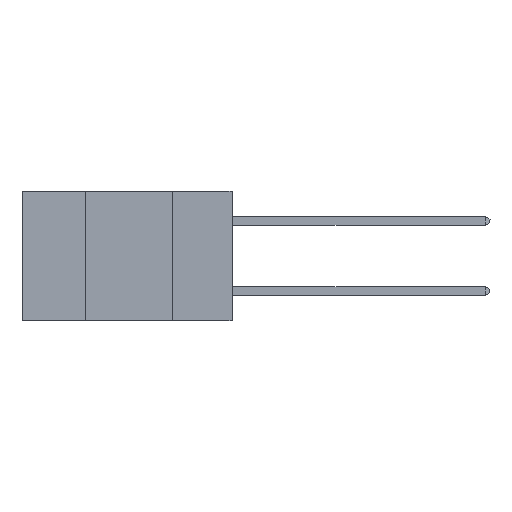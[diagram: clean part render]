
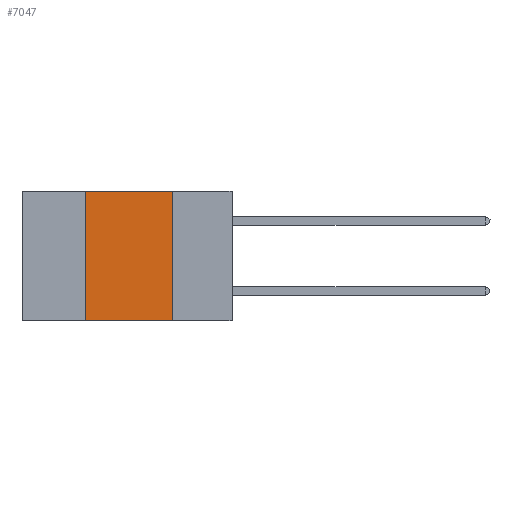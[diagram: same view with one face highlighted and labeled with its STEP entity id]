
A CAD part, left-side view. The second image highlights one B-rep face of the part: STEP entity #7047.
In plain terms, the highlighted planar face has unit normal (-1, 0, 0).
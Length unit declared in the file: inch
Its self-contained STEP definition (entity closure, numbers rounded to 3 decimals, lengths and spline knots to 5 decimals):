
#255 = VECTOR ( 'NONE', #21321, 39.37008 ) ;
#381 = ORIENTED_EDGE ( 'NONE', *, *, #14641, .F. ) ;
#794 = ORIENTED_EDGE ( 'NONE', *, *, #16202, .T. ) ;
#1057 = CARTESIAN_POINT ( 'NONE',  ( 0., 0.6, -0.37 ) ) ;
#1485 = EDGE_CURVE ( 'NONE', #5787, #17818, #10814, .T. ) ;
#2426 = ORIENTED_EDGE ( 'NONE', *, *, #1485, .F. ) ;
#2644 = CARTESIAN_POINT ( 'NONE',  ( 0., 0.42, 0. ) ) ;
#4587 = LINE ( 'NONE', #1057, #13866 ) ;
#5331 = PLANE ( 'NONE',  #9582 ) ;
#5787 = VERTEX_POINT ( 'NONE', #9061 ) ;
#5947 = CARTESIAN_POINT ( 'NONE',  ( 0., 0.6, 0. ) ) ;
#7047 = ADVANCED_FACE ( 'NONE', ( #14817 ), #5331, .F. ) ;
#7091 = DIRECTION ( 'NONE',  ( 0., 0., -1. ) ) ;
#7653 = EDGE_CURVE ( 'NONE', #10540, #5787, #18887, .T. ) ;
#8600 = VECTOR ( 'NONE', #21697, 39.37008 ) ;
#8654 = DIRECTION ( 'NONE',  ( 1., 0., 0. ) ) ;
#9061 = CARTESIAN_POINT ( 'NONE',  ( 0., 0.42, 0. ) ) ;
#9582 = AXIS2_PLACEMENT_3D ( 'NONE', #19176, #8654, #7091 ) ;
#10540 = VERTEX_POINT ( 'NONE', #14940 ) ;
#10814 = LINE ( 'NONE', #5947, #18385 ) ;
#11047 = CARTESIAN_POINT ( 'NONE',  ( 0., 0.17, 0. ) ) ;
#12334 = EDGE_LOOP ( 'NONE', ( #381, #2426, #12465, #794 ) ) ;
#12465 = ORIENTED_EDGE ( 'NONE', *, *, #7653, .F. ) ;
#13224 = DIRECTION ( 'NONE',  ( 0., -1., 0. ) ) ;
#13866 = VECTOR ( 'NONE', #13224, 39.37008 ) ;
#14641 = EDGE_CURVE ( 'NONE', #17818, #15252, #19859, .T. ) ;
#14817 = FACE_OUTER_BOUND ( 'NONE', #12334, .T. ) ;
#14940 = CARTESIAN_POINT ( 'NONE',  ( 0., 0.42, -0.37 ) ) ;
#15252 = VERTEX_POINT ( 'NONE', #19696 ) ;
#16202 = EDGE_CURVE ( 'NONE', #10540, #15252, #4587, .T. ) ;
#17818 = VERTEX_POINT ( 'NONE', #11047 ) ;
#18082 = DIRECTION ( 'NONE',  ( 0., -1., 0. ) ) ;
#18385 = VECTOR ( 'NONE', #18082, 39.37008 ) ;
#18887 = LINE ( 'NONE', #2644, #8600 ) ;
#19176 = CARTESIAN_POINT ( 'NONE',  ( 0., 0.6, 0. ) ) ;
#19696 = CARTESIAN_POINT ( 'NONE',  ( 0., 0.17, -0.37 ) ) ;
#19859 = LINE ( 'NONE', #21400, #255 ) ;
#21321 = DIRECTION ( 'NONE',  ( 0., 0., -1. ) ) ;
#21400 = CARTESIAN_POINT ( 'NONE',  ( 0., 0.17, 0. ) ) ;
#21697 = DIRECTION ( 'NONE',  ( 0., 0., 1. ) ) ;
